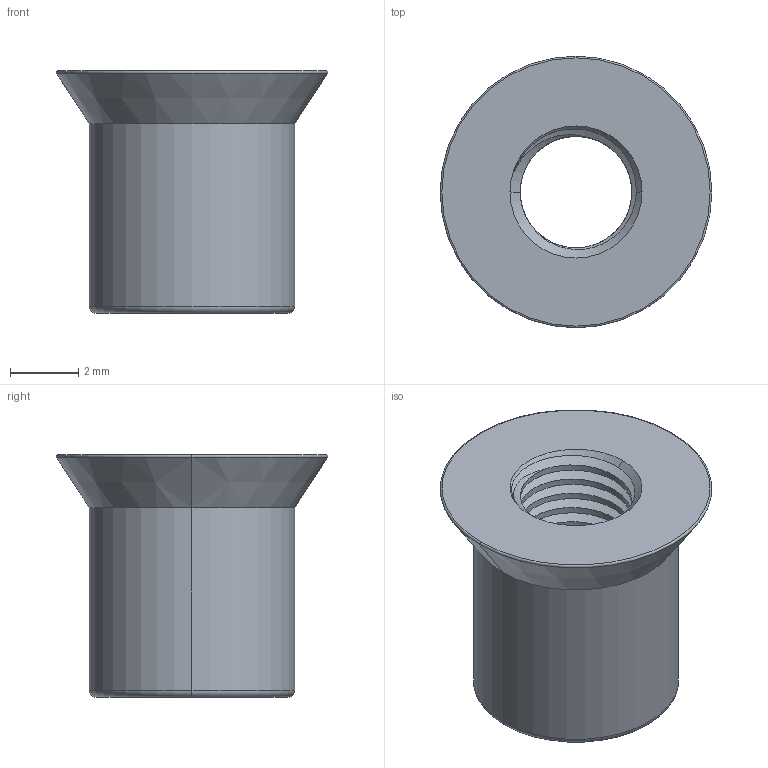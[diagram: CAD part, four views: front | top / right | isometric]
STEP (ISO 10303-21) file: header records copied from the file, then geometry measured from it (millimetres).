
FILE_DESCRIPTION (( 'STEP AP214' ), '1' );
FILE_NAME ('Zentrierstück.STEP', '2013-07-30T15:10:54', ( 'Asher' ), ( '' ), 'SwSTEP 2.0', 'SolidWorks 2013', '' );
FILE_SCHEMA (( 'AUTOMOTIVE_DESIGN' ));
Length unit declared in the file: millimetre
Products named in the file (1): Zentrierstück
Bounding box: 7.93 x 7.93 x 7.09 mm (x, y, z)
Volume: 145.4 mm3; surface area: 314.7 mm2
Topology: 1 solids, 1 shells, 41 faces, 106 edges, 68 vertices
Faces by surface type: cylinder 26, cone 6, torus 4, plane 3, bspline 2
Entity records: 2169 total; most frequent: CARTESIAN_POINT 1254, ORIENTED_EDGE 212, DIRECTION 163, EDGE_CURVE 106, VERTEX_POINT 68, AXIS2_PLACEMENT_3D 66, EDGE_LOOP 44, ADVANCED_FACE 41
